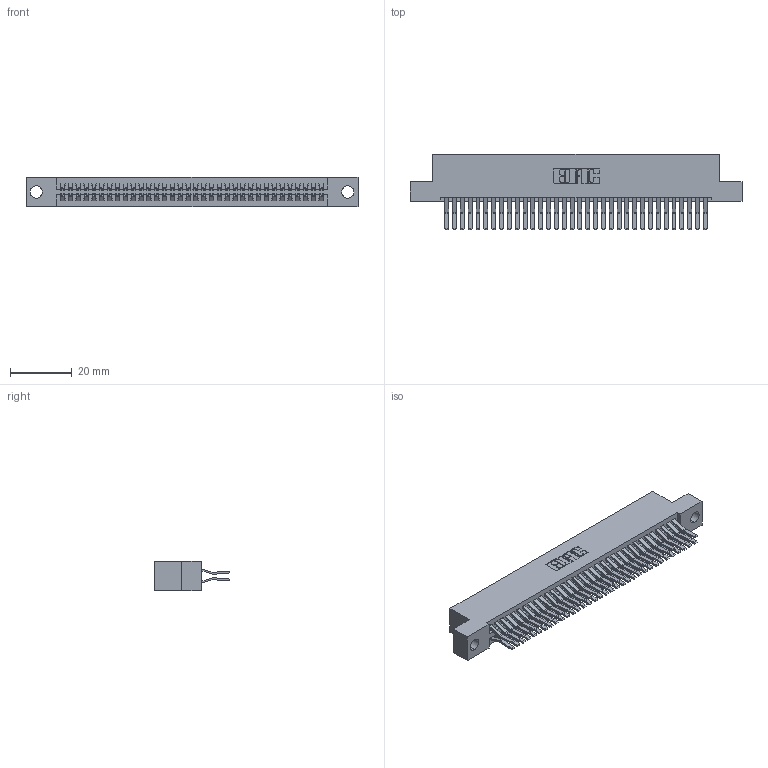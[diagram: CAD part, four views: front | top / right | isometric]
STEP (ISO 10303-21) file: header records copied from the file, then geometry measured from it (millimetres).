
FILE_DESCRIPTION (( 'STEP AP203' ), '1' );
FILE_NAME ('345-068-560-204.STEP', '2018-09-30T16:05:38', ( '' ), ( '' ), 'SwSTEP 2.0', 'SolidWorks 2016', '' );
FILE_SCHEMA (( 'CONFIG_CONTROL_DESIGN' ));
Length unit declared in the file: inch
Products named in the file (3): 345 Part_Flush Mounting Lugs - 0.156 Dia-TH; 345-292-001_560 Tail; 345-068-560-204
Assembly tree (69 placements, depth 2):
  345-068-560-204
    345 Part_Flush Mounting Lugs - 0.156 Dia-TH
    345-292-001_560 Tail  x68
Bounding box: 107.57 x 24.45 x 9.4 mm (x, y, z)
Volume: 10733 mm3; surface area: 16671.7 mm2
Topology: 69 solids, 69 shells, 3662 faces, 10881 edges, 7162 vertices
Faces by surface type: plane 2324, cylinder 1338
Entity records: 27845 total; most frequent: CARTESIAN_POINT 4676, ORIENTED_EDGE 4610, DIRECTION 4137, EDGE_CURVE 2305, VECTOR 2033, LINE 2033, VERTEX_POINT 1534, AXIS2_PLACEMENT_3D 1052
